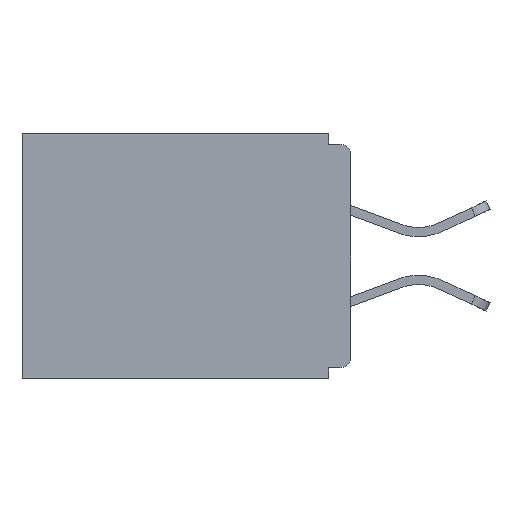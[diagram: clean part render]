
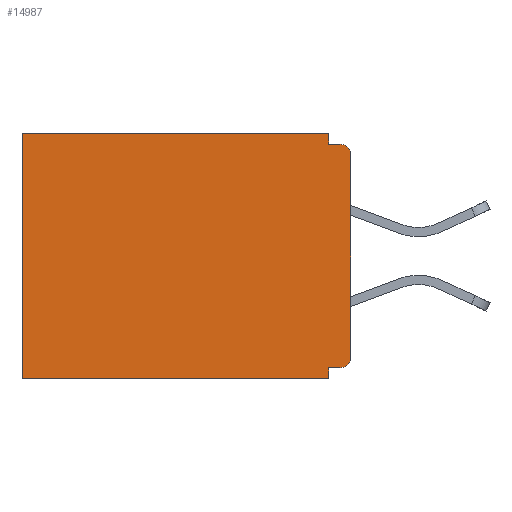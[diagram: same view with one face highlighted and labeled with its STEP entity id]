
A CAD part, left-side view. The second image highlights one B-rep face of the part: STEP entity #14987.
In plain terms, the highlighted planar face has unit normal (-1, 0, 0).
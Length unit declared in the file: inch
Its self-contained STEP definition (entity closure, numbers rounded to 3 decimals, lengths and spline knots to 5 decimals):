
#225 = ORIENTED_EDGE ( 'NONE', *, *, #582, .F. ) ;
#429 = VECTOR ( 'NONE', #21291, 39.37008 ) ;
#582 = EDGE_CURVE ( 'NONE', #7121, #13113, #1861, .T. ) ;
#1315 = CARTESIAN_POINT ( 'NONE',  ( 0.298, 0., -0.313 ) ) ;
#1375 = VECTOR ( 'NONE', #4413, 39.37008 ) ;
#1861 = LINE ( 'NONE', #17081, #18823 ) ;
#2249 = DIRECTION ( 'NONE',  ( 0., 1., 0. ) ) ;
#2332 = CARTESIAN_POINT ( 'NONE',  ( 0.298, 0.015, -0.03 ) ) ;
#2834 = ORIENTED_EDGE ( 'NONE', *, *, #16724, .F. ) ;
#2957 = ORIENTED_EDGE ( 'NONE', *, *, #12246, .T. ) ;
#3020 = CARTESIAN_POINT ( 'NONE',  ( 0.298, 0.015, -0.313 ) ) ;
#3398 = EDGE_CURVE ( 'NONE', #22807, #7121, #18716, .T. ) ;
#3630 = VERTEX_POINT ( 'NONE', #7483 ) ;
#3974 = VECTOR ( 'NONE', #10136, 39.37008 ) ;
#4117 = AXIS2_PLACEMENT_3D ( 'NONE', #20489, #20811, #13409 ) ;
#4293 = VERTEX_POINT ( 'NONE', #1315 ) ;
#4413 = DIRECTION ( 'NONE',  ( 0., 0., -1. ) ) ;
#4611 = ORIENTED_EDGE ( 'NONE', *, *, #5663, .F. ) ;
#5504 = VECTOR ( 'NONE', #14433, 39.37008 ) ;
#5663 = EDGE_CURVE ( 'NONE', #20905, #6170, #13627, .T. ) ;
#5716 = EDGE_CURVE ( 'NONE', #23444, #4293, #15376, .T. ) ;
#6007 = EDGE_LOOP ( 'NONE', ( #7059, #4611, #14133, #2957, #22563, #225, #22319, #2834, #13368, #20488 ) ) ;
#6107 = DIRECTION ( 'NONE',  ( -1., 0., 0. ) ) ;
#6170 = VERTEX_POINT ( 'NONE', #22860 ) ;
#6971 = LINE ( 'NONE', #8055, #1375 ) ;
#7059 = ORIENTED_EDGE ( 'NONE', *, *, #7524, .T. ) ;
#7121 = VERTEX_POINT ( 'NONE', #24070 ) ;
#7483 = CARTESIAN_POINT ( 'NONE',  ( 0.298, 0.015, -0.328 ) ) ;
#7524 = EDGE_CURVE ( 'NONE', #23444, #6170, #8940, .T. ) ;
#8055 = CARTESIAN_POINT ( 'NONE',  ( 0.298, 0.46, 0. ) ) ;
#8194 = EDGE_CURVE ( 'NONE', #3630, #4293, #8895, .T. ) ;
#8416 = LINE ( 'NONE', #22993, #3974 ) ;
#8895 = CIRCLE ( 'NONE', #22856, 0.015 ) ;
#8940 = CIRCLE ( 'NONE', #18281, 0.015 ) ;
#9257 = VERTEX_POINT ( 'NONE', #16684 ) ;
#9810 = VECTOR ( 'NONE', #17483, 39.37008 ) ;
#9938 = CARTESIAN_POINT ( 'NONE',  ( 0.298, 0., 0. ) ) ;
#10033 = VECTOR ( 'NONE', #18354, 39.37008 ) ;
#10136 = DIRECTION ( 'NONE',  ( 0., 0., -1. ) ) ;
#12246 = EDGE_CURVE ( 'NONE', #9257, #20719, #18370, .T. ) ;
#12577 = CARTESIAN_POINT ( 'NONE',  ( 0.298, 0., -0.328 ) ) ;
#12749 = CARTESIAN_POINT ( 'NONE',  ( 0.298, 0., -0.03 ) ) ;
#13113 = VERTEX_POINT ( 'NONE', #23608 ) ;
#13364 = EDGE_CURVE ( 'NONE', #20719, #13113, #6971, .T. ) ;
#13368 = ORIENTED_EDGE ( 'NONE', *, *, #8194, .T. ) ;
#13409 = DIRECTION ( 'NONE',  ( 0., 0., -1. ) ) ;
#13627 = LINE ( 'NONE', #21451, #9810 ) ;
#14133 = ORIENTED_EDGE ( 'NONE', *, *, #20292, .F. ) ;
#14177 = DIRECTION ( 'NONE',  ( -1., 0., 0. ) ) ;
#14419 = DIRECTION ( 'NONE',  ( 0., 0., -1. ) ) ;
#14433 = DIRECTION ( 'NONE',  ( 0., 1., 0. ) ) ;
#14987 = ADVANCED_FACE ( 'NONE', ( #18556 ), #18531, .F. ) ;
#15376 = LINE ( 'NONE', #9938, #429 ) ;
#16684 = CARTESIAN_POINT ( 'NONE',  ( 0.298, 0.031, 0. ) ) ;
#16724 = EDGE_CURVE ( 'NONE', #3630, #22807, #19967, .T. ) ;
#17081 = CARTESIAN_POINT ( 'NONE',  ( 0.298, 0., -0.343 ) ) ;
#17483 = DIRECTION ( 'NONE',  ( 0., -1., 0. ) ) ;
#17849 = DIRECTION ( 'NONE',  ( 0., 0., -1. ) ) ;
#18281 = AXIS2_PLACEMENT_3D ( 'NONE', #2332, #6107, #19184 ) ;
#18342 = CARTESIAN_POINT ( 'NONE',  ( 0.298, 0., 0. ) ) ;
#18354 = DIRECTION ( 'NONE',  ( 0., 1., 0. ) ) ;
#18370 = LINE ( 'NONE', #18342, #5504 ) ;
#18531 = PLANE ( 'NONE',  #4117 ) ;
#18556 = FACE_OUTER_BOUND ( 'NONE', #6007, .T. ) ;
#18716 = LINE ( 'NONE', #22103, #19311 ) ;
#18823 = VECTOR ( 'NONE', #2249, 39.37008 ) ;
#19184 = DIRECTION ( 'NONE',  ( 0., 0., -1. ) ) ;
#19311 = VECTOR ( 'NONE', #14419, 39.37008 ) ;
#19917 = CARTESIAN_POINT ( 'NONE',  ( 0.298, 0.031, -0.015 ) ) ;
#19967 = LINE ( 'NONE', #12577, #10033 ) ;
#20292 = EDGE_CURVE ( 'NONE', #9257, #20905, #8416, .T. ) ;
#20351 = CARTESIAN_POINT ( 'NONE',  ( 0.298, 0.031, -0.328 ) ) ;
#20422 = CARTESIAN_POINT ( 'NONE',  ( 0.298, 0.46, 0. ) ) ;
#20488 = ORIENTED_EDGE ( 'NONE', *, *, #5716, .F. ) ;
#20489 = CARTESIAN_POINT ( 'NONE',  ( 0.298, 0., 0. ) ) ;
#20719 = VERTEX_POINT ( 'NONE', #20422 ) ;
#20811 = DIRECTION ( 'NONE',  ( 1., 0., 0. ) ) ;
#20905 = VERTEX_POINT ( 'NONE', #19917 ) ;
#21291 = DIRECTION ( 'NONE',  ( 0., 0., -1. ) ) ;
#21451 = CARTESIAN_POINT ( 'NONE',  ( 0.298, 0., -0.015 ) ) ;
#22103 = CARTESIAN_POINT ( 'NONE',  ( 0.298, 0.031, -0.343 ) ) ;
#22319 = ORIENTED_EDGE ( 'NONE', *, *, #3398, .F. ) ;
#22563 = ORIENTED_EDGE ( 'NONE', *, *, #13364, .T. ) ;
#22807 = VERTEX_POINT ( 'NONE', #20351 ) ;
#22856 = AXIS2_PLACEMENT_3D ( 'NONE', #3020, #14177, #17849 ) ;
#22860 = CARTESIAN_POINT ( 'NONE',  ( 0.298, 0.015, -0.015 ) ) ;
#22993 = CARTESIAN_POINT ( 'NONE',  ( 0.298, 0.031, -0.343 ) ) ;
#23444 = VERTEX_POINT ( 'NONE', #12749 ) ;
#23608 = CARTESIAN_POINT ( 'NONE',  ( 0.298, 0.46, -0.343 ) ) ;
#24070 = CARTESIAN_POINT ( 'NONE',  ( 0.298, 0.031, -0.343 ) ) ;
